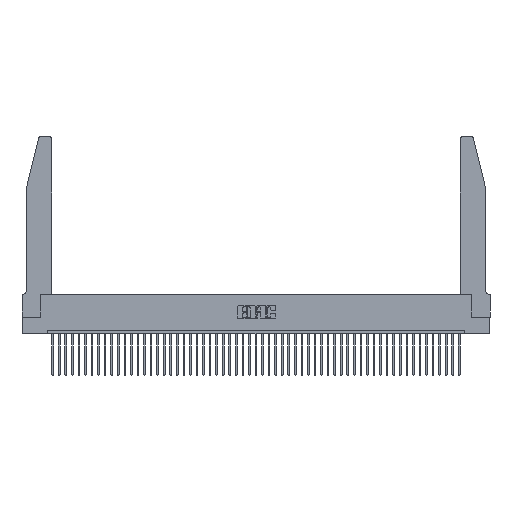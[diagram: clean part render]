
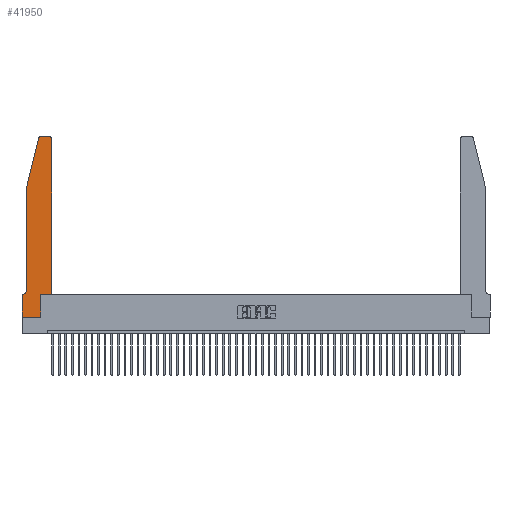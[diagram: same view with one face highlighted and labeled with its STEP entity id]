
A CAD part, top view. The second image highlights one B-rep face of the part: STEP entity #41950.
In plain terms, the highlighted planar face has unit normal (0, 0, 1).
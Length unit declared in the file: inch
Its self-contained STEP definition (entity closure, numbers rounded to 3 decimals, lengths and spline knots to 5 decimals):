
#339 = ORIENTED_EDGE ( 'NONE', *, *, #11633, .T. ) ;
#740 = CARTESIAN_POINT ( 'NONE',  ( 0.4505, 0.35, 0.37 ) ) ;
#984 = LINE ( 'NONE', #19355, #2279 ) ;
#1946 = VERTEX_POINT ( 'NONE', #5364 ) ;
#2279 = VECTOR ( 'NONE', #47947, 39.37008 ) ;
#2423 = LINE ( 'NONE', #33201, #23305 ) ;
#2614 = CARTESIAN_POINT ( 'NONE',  ( 0.2865, 0.35, 0.37 ) ) ;
#2661 = CARTESIAN_POINT ( 'NONE',  ( 0.4205, 2.72, 0.37 ) ) ;
#2861 = DIRECTION ( 'NONE',  ( 1., 0., 0. ) ) ;
#3569 = ORIENTED_EDGE ( 'NONE', *, *, #32722, .T. ) ;
#3659 = EDGE_CURVE ( 'NONE', #10489, #27710, #5191, .T. ) ;
#3717 = LINE ( 'NONE', #17099, #43038 ) ;
#4027 = VECTOR ( 'NONE', #15605, 39.37008 ) ;
#4068 = VECTOR ( 'NONE', #13662, 39.37008 ) ;
#4355 = ORIENTED_EDGE ( 'NONE', *, *, #25361, .T. ) ;
#4637 = CARTESIAN_POINT ( 'NONE',  ( 0.4205, 2.75, 0.37 ) ) ;
#5050 = AXIS2_PLACEMENT_3D ( 'NONE', #2661, #40880, #44681 ) ;
#5191 = LINE ( 'NONE', #21643, #4027 ) ;
#5364 = CARTESIAN_POINT ( 'NONE',  ( 0.25487, 2.72718, 0.37 ) ) ;
#5525 = VERTEX_POINT ( 'NONE', #41405 ) ;
#5554 = CARTESIAN_POINT ( 'NONE',  ( 0.0055, 0.35, 0.37 ) ) ;
#5965 = CARTESIAN_POINT ( 'NONE',  ( 0.284, 2.72, 0.37 ) ) ;
#6310 = VECTOR ( 'NONE', #12033, 39.37008 ) ;
#6916 = LINE ( 'NONE', #2614, #7508 ) ;
#7388 = CARTESIAN_POINT ( 'NONE',  ( 0.0055, 0.42, 0.37 ) ) ;
#7508 = VECTOR ( 'NONE', #18654, 39.37008 ) ;
#7659 = ORIENTED_EDGE ( 'NONE', *, *, #15812, .T. ) ;
#9103 = DIRECTION ( 'NONE',  ( 1., 0., 0. ) ) ;
#10159 = ORIENTED_EDGE ( 'NONE', *, *, #19855, .T. ) ;
#10368 = PLANE ( 'NONE',  #14120 ) ;
#10489 = VERTEX_POINT ( 'NONE', #47358 ) ;
#11493 = CIRCLE ( 'NONE', #41462, 0.03 ) ;
#11633 = EDGE_CURVE ( 'NONE', #15876, #5525, #2423, .T. ) ;
#11793 = ORIENTED_EDGE ( 'NONE', *, *, #34353, .T. ) ;
#12033 = DIRECTION ( 'NONE',  ( 0., 1., 0. ) ) ;
#12575 = LINE ( 'NONE', #19526, #48407 ) ;
#13662 = DIRECTION ( 'NONE',  ( 0., -1., 0. ) ) ;
#14120 = AXIS2_PLACEMENT_3D ( 'NONE', #21775, #21931, #2861 ) ;
#14234 = ORIENTED_EDGE ( 'NONE', *, *, #14406, .T. ) ;
#14274 = LINE ( 'NONE', #17360, #4068 ) ;
#14406 = EDGE_CURVE ( 'NONE', #5525, #41435, #14274, .T. ) ;
#14731 = CARTESIAN_POINT ( 'NONE',  ( 0.284, 2.75, 0.37 ) ) ;
#15212 = FACE_OUTER_BOUND ( 'NONE', #23949, .T. ) ;
#15605 = DIRECTION ( 'NONE',  ( 0., -1., 0. ) ) ;
#15706 = VERTEX_POINT ( 'NONE', #23888 ) ;
#15786 = LINE ( 'NONE', #39148, #6310 ) ;
#15812 = EDGE_CURVE ( 'NONE', #1946, #10489, #3717, .T. ) ;
#15876 = VERTEX_POINT ( 'NONE', #5554 ) ;
#16937 = ORIENTED_EDGE ( 'NONE', *, *, #24131, .T. ) ;
#17099 = CARTESIAN_POINT ( 'NONE',  ( 0.0755, 2., 0.37 ) ) ;
#17360 = CARTESIAN_POINT ( 'NONE',  ( 0., 0., 0.37 ) ) ;
#17584 = CARTESIAN_POINT ( 'NONE',  ( 0.2865, 0.35, 0.37 ) ) ;
#17636 = CIRCLE ( 'NONE', #5050, 0.03 ) ;
#17751 = CARTESIAN_POINT ( 'NONE',  ( 0.2605, 2.75, 0.37 ) ) ;
#18654 = DIRECTION ( 'NONE',  ( 0., 1., 0. ) ) ;
#19355 = CARTESIAN_POINT ( 'NONE',  ( 0.4505, 0.35, 0.37 ) ) ;
#19397 = DIRECTION ( 'NONE',  ( 1., 0., 0. ) ) ;
#19526 = CARTESIAN_POINT ( 'NONE',  ( 0., 0., 0.37 ) ) ;
#19855 = EDGE_CURVE ( 'NONE', #29706, #37133, #15786, .T. ) ;
#21643 = CARTESIAN_POINT ( 'NONE',  ( 0.0755, 2., 0.37 ) ) ;
#21775 = CARTESIAN_POINT ( 'NONE',  ( 0., 0.35, 0.37 ) ) ;
#21931 = DIRECTION ( 'NONE',  ( 0., 0., 1. ) ) ;
#22063 = DIRECTION ( 'NONE',  ( -1., 0., 0. ) ) ;
#23305 = VECTOR ( 'NONE', #22063, 39.37008 ) ;
#23888 = CARTESIAN_POINT ( 'NONE',  ( 0.2865, 0., 0.37 ) ) ;
#23949 = EDGE_LOOP ( 'NONE', ( #16937, #42985, #7659, #40105, #3569, #339, #14234, #4355, #11793, #32746, #10159, #39109 ) ) ;
#24131 = EDGE_CURVE ( 'NONE', #47091, #25902, #46688, .T. ) ;
#25361 = EDGE_CURVE ( 'NONE', #41435, #15706, #12575, .T. ) ;
#25808 = VERTEX_POINT ( 'NONE', #17584 ) ;
#25902 = VERTEX_POINT ( 'NONE', #14731 ) ;
#27574 = VECTOR ( 'NONE', #37475, 39.37008 ) ;
#27710 = VERTEX_POINT ( 'NONE', #29046 ) ;
#27804 = AXIS2_PLACEMENT_3D ( 'NONE', #7388, #41570, #45369 ) ;
#29046 = CARTESIAN_POINT ( 'NONE',  ( 0.0755, 0.42, 0.37 ) ) ;
#29706 = VERTEX_POINT ( 'NONE', #740 ) ;
#32722 = EDGE_CURVE ( 'NONE', #27710, #15876, #41560, .T. ) ;
#32746 = ORIENTED_EDGE ( 'NONE', *, *, #38077, .T. ) ;
#33201 = CARTESIAN_POINT ( 'NONE',  ( 0.0755, 0.35, 0.37 ) ) ;
#34353 = EDGE_CURVE ( 'NONE', #15706, #25808, #6916, .T. ) ;
#37133 = VERTEX_POINT ( 'NONE', #39590 ) ;
#37475 = DIRECTION ( 'NONE',  ( -1., 0., 0. ) ) ;
#38077 = EDGE_CURVE ( 'NONE', #25808, #29706, #984, .T. ) ;
#39109 = ORIENTED_EDGE ( 'NONE', *, *, #40514, .T. ) ;
#39148 = CARTESIAN_POINT ( 'NONE',  ( 0.4505, 0.35, 0.37 ) ) ;
#39590 = CARTESIAN_POINT ( 'NONE',  ( 0.4505, 2.72, 0.37 ) ) ;
#40105 = ORIENTED_EDGE ( 'NONE', *, *, #3659, .T. ) ;
#40514 = EDGE_CURVE ( 'NONE', #37133, #47091, #17636, .T. ) ;
#40880 = DIRECTION ( 'NONE',  ( 0., 0., 1. ) ) ;
#41405 = CARTESIAN_POINT ( 'NONE',  ( 0., 0.35, 0.37 ) ) ;
#41435 = VERTEX_POINT ( 'NONE', #47179 ) ;
#41462 = AXIS2_PLACEMENT_3D ( 'NONE', #5965, #47589, #9103 ) ;
#41560 = CIRCLE ( 'NONE', #27804, 0.07 ) ;
#41570 = DIRECTION ( 'NONE',  ( 0., 0., -1. ) ) ;
#41950 = ADVANCED_FACE ( 'NONE', ( #15212 ), #10368, .T. ) ;
#42985 = ORIENTED_EDGE ( 'NONE', *, *, #47861, .T. ) ;
#43038 = VECTOR ( 'NONE', #43753, 39.37008 ) ;
#43753 = DIRECTION ( 'NONE',  ( -0.239, -0.971, 0. ) ) ;
#44681 = DIRECTION ( 'NONE',  ( 1., 0., 0. ) ) ;
#45369 = DIRECTION ( 'NONE',  ( -1., 0., 0. ) ) ;
#46688 = LINE ( 'NONE', #17751, #27574 ) ;
#47091 = VERTEX_POINT ( 'NONE', #4637 ) ;
#47179 = CARTESIAN_POINT ( 'NONE',  ( 0., 0., 0.37 ) ) ;
#47358 = CARTESIAN_POINT ( 'NONE',  ( 0.0755, 2., 0.37 ) ) ;
#47589 = DIRECTION ( 'NONE',  ( 0., 0., 1. ) ) ;
#47861 = EDGE_CURVE ( 'NONE', #25902, #1946, #11493, .T. ) ;
#47947 = DIRECTION ( 'NONE',  ( 1., 0., 0. ) ) ;
#48407 = VECTOR ( 'NONE', #19397, 39.37008 ) ;
